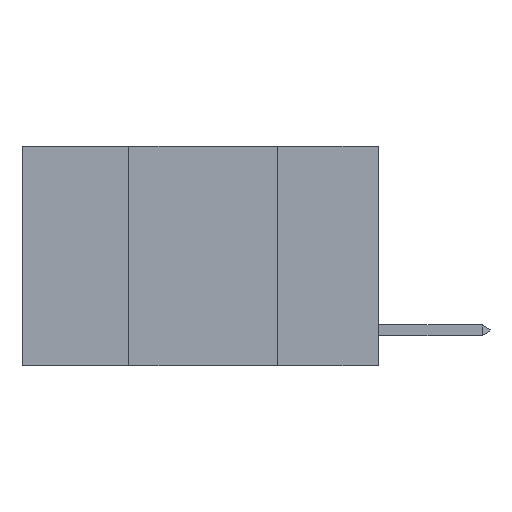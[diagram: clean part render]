
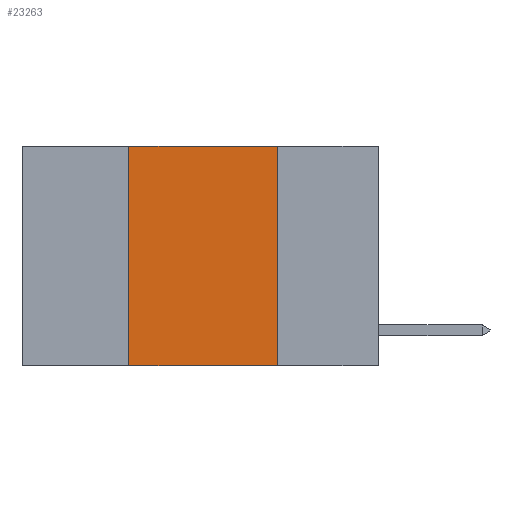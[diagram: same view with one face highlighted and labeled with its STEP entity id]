
A CAD part, left-side view. The second image highlights one B-rep face of the part: STEP entity #23263.
In plain terms, the highlighted planar face has unit normal (-1, 0, 0).
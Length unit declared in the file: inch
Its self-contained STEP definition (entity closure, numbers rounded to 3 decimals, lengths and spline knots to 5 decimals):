
#574 = LINE ( 'NONE', #1816, #4853 ) ;
#1134 = VERTEX_POINT ( 'NONE', #21761 ) ;
#1437 = ORIENTED_EDGE ( 'NONE', *, *, #6032, .T. ) ;
#1526 = CARTESIAN_POINT ( 'NONE',  ( 0., 0.6, 0. ) ) ;
#1739 = LINE ( 'NONE', #5626, #15129 ) ;
#1816 = CARTESIAN_POINT ( 'NONE',  ( 0., 0.17, 0. ) ) ;
#2713 = DIRECTION ( 'NONE',  ( 0., 0., -1. ) ) ;
#4853 = VECTOR ( 'NONE', #16340, 39.37008 ) ;
#5213 = DIRECTION ( 'NONE',  ( 0., -1., 0. ) ) ;
#5626 = CARTESIAN_POINT ( 'NONE',  ( 0., 0.42, 0. ) ) ;
#5797 = EDGE_CURVE ( 'NONE', #10874, #1134, #574, .T. ) ;
#6032 = EDGE_CURVE ( 'NONE', #8071, #1134, #14813, .T. ) ;
#6517 = CARTESIAN_POINT ( 'NONE',  ( 0., 0.42, -0.37 ) ) ;
#7236 = VERTEX_POINT ( 'NONE', #9719 ) ;
#7237 = VECTOR ( 'NONE', #5213, 39.37008 ) ;
#7408 = FACE_OUTER_BOUND ( 'NONE', #17757, .T. ) ;
#7905 = CARTESIAN_POINT ( 'NONE',  ( 0., 0.6, -0.37 ) ) ;
#8071 = VERTEX_POINT ( 'NONE', #6517 ) ;
#9719 = CARTESIAN_POINT ( 'NONE',  ( 0., 0.42, 0. ) ) ;
#10544 = AXIS2_PLACEMENT_3D ( 'NONE', #13550, #13622, #2713 ) ;
#10597 = EDGE_CURVE ( 'NONE', #7236, #10874, #21607, .T. ) ;
#10651 = ORIENTED_EDGE ( 'NONE', *, *, #5797, .F. ) ;
#10874 = VERTEX_POINT ( 'NONE', #11370 ) ;
#11370 = CARTESIAN_POINT ( 'NONE',  ( 0., 0.17, 0. ) ) ;
#13550 = CARTESIAN_POINT ( 'NONE',  ( 0., 0.6, 0. ) ) ;
#13622 = DIRECTION ( 'NONE',  ( 1., 0., 0. ) ) ;
#14813 = LINE ( 'NONE', #7905, #20138 ) ;
#15129 = VECTOR ( 'NONE', #20094, 39.37008 ) ;
#16340 = DIRECTION ( 'NONE',  ( 0., 0., -1. ) ) ;
#17757 = EDGE_LOOP ( 'NONE', ( #10651, #23178, #19588, #1437 ) ) ;
#18694 = DIRECTION ( 'NONE',  ( 0., -1., 0. ) ) ;
#19588 = ORIENTED_EDGE ( 'NONE', *, *, #21695, .F. ) ;
#20094 = DIRECTION ( 'NONE',  ( 0., 0., 1. ) ) ;
#20138 = VECTOR ( 'NONE', #18694, 39.37008 ) ;
#21607 = LINE ( 'NONE', #1526, #7237 ) ;
#21695 = EDGE_CURVE ( 'NONE', #8071, #7236, #1739, .T. ) ;
#21761 = CARTESIAN_POINT ( 'NONE',  ( 0., 0.17, -0.37 ) ) ;
#22521 = PLANE ( 'NONE',  #10544 ) ;
#23178 = ORIENTED_EDGE ( 'NONE', *, *, #10597, .F. ) ;
#23263 = ADVANCED_FACE ( 'NONE', ( #7408 ), #22521, .F. ) ;
